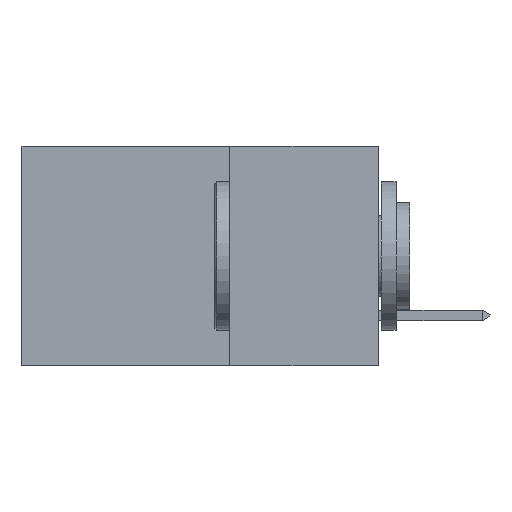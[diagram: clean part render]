
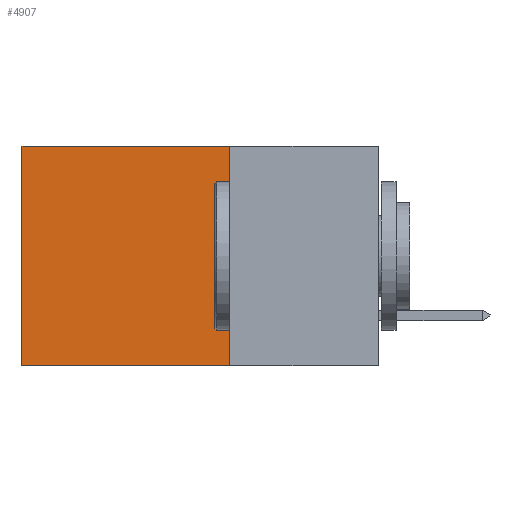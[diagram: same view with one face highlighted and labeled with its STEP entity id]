
A CAD part, left-side view. The second image highlights one B-rep face of the part: STEP entity #4907.
In plain terms, the highlighted planar face has unit normal (-1, 0, 0).
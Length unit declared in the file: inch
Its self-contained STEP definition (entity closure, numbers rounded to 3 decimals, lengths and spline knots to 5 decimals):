
#312 = ORIENTED_EDGE ( 'NONE', *, *, #15719, .T. ) ;
#988 = LINE ( 'NONE', #1593, #12162 ) ;
#1284 = VERTEX_POINT ( 'NONE', #17355 ) ;
#1475 = DIRECTION ( 'NONE',  ( 0., 0., -1. ) ) ;
#1593 = CARTESIAN_POINT ( 'NONE',  ( 0.298, 0.25, -0.37 ) ) ;
#1738 = ORIENTED_EDGE ( 'NONE', *, *, #10212, .T. ) ;
#1867 = DIRECTION ( 'NONE',  ( 0., 0., -1. ) ) ;
#3340 = FACE_OUTER_BOUND ( 'NONE', #16386, .T. ) ;
#3779 = CARTESIAN_POINT ( 'NONE',  ( 0.298, 0.25, 0. ) ) ;
#4798 = EDGE_CURVE ( 'NONE', #6094, #16782, #16965, .T. ) ;
#4907 = ADVANCED_FACE ( 'NONE', ( #3340 ), #12743, .F. ) ;
#5392 = VECTOR ( 'NONE', #1867, 39.37008 ) ;
#5699 = VERTEX_POINT ( 'NONE', #17073 ) ;
#6094 = VERTEX_POINT ( 'NONE', #14501 ) ;
#6746 = ORIENTED_EDGE ( 'NONE', *, *, #4798, .F. ) ;
#7260 = DIRECTION ( 'NONE',  ( 1., 0., 0. ) ) ;
#7746 = AXIS2_PLACEMENT_3D ( 'NONE', #16748, #7260, #1475 ) ;
#8391 = DIRECTION ( 'NONE',  ( 0., 1., 0. ) ) ;
#8919 = ORIENTED_EDGE ( 'NONE', *, *, #16932, .F. ) ;
#10212 = EDGE_CURVE ( 'NONE', #1284, #5699, #17714, .T. ) ;
#11575 = VECTOR ( 'NONE', #13614, 39.37008 ) ;
#11759 = VECTOR ( 'NONE', #16271, 39.37008 ) ;
#12162 = VECTOR ( 'NONE', #8391, 39.37008 ) ;
#12743 = PLANE ( 'NONE',  #7746 ) ;
#13614 = DIRECTION ( 'NONE',  ( 0., 1., 0. ) ) ;
#14501 = CARTESIAN_POINT ( 'NONE',  ( 0.298, 0.25, 0. ) ) ;
#14895 = CARTESIAN_POINT ( 'NONE',  ( 0.298, 0.25, 0. ) ) ;
#15692 = LINE ( 'NONE', #14895, #11575 ) ;
#15719 = EDGE_CURVE ( 'NONE', #6094, #1284, #15692, .T. ) ;
#16060 = CARTESIAN_POINT ( 'NONE',  ( 0.298, 0.25, -0.37 ) ) ;
#16271 = DIRECTION ( 'NONE',  ( 0., 0., -1. ) ) ;
#16386 = EDGE_LOOP ( 'NONE', ( #1738, #8919, #6746, #312 ) ) ;
#16748 = CARTESIAN_POINT ( 'NONE',  ( 0.298, 0.25, 0. ) ) ;
#16782 = VERTEX_POINT ( 'NONE', #16060 ) ;
#16884 = CARTESIAN_POINT ( 'NONE',  ( 0.298, 0.6, 0. ) ) ;
#16932 = EDGE_CURVE ( 'NONE', #16782, #5699, #988, .T. ) ;
#16965 = LINE ( 'NONE', #3779, #11759 ) ;
#17073 = CARTESIAN_POINT ( 'NONE',  ( 0.298, 0.6, -0.37 ) ) ;
#17355 = CARTESIAN_POINT ( 'NONE',  ( 0.298, 0.6, 0. ) ) ;
#17714 = LINE ( 'NONE', #16884, #5392 ) ;
